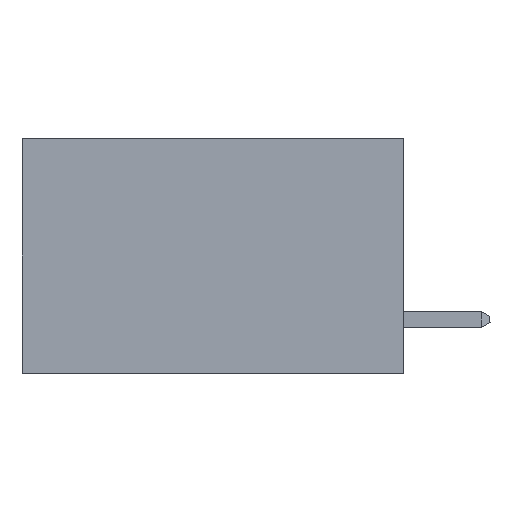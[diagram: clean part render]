
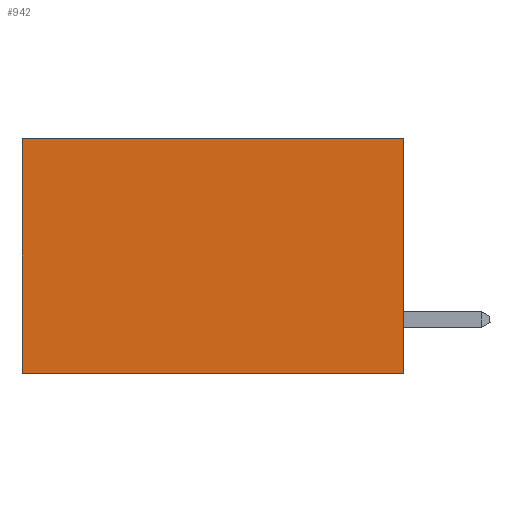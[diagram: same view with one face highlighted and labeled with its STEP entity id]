
A CAD part, left-side view. The second image highlights one B-rep face of the part: STEP entity #942.
In plain terms, the highlighted planar face has unit normal (-1, 0, 0).
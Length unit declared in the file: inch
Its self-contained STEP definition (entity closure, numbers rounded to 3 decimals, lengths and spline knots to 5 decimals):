
#180 = LINE ( 'NONE', #2519, #1146 ) ;
#942 = ADVANCED_FACE ( 'NONE', ( #18578 ), #19189, .F. ) ;
#993 = ORIENTED_EDGE ( 'NONE', *, *, #8523, .F. ) ;
#1146 = VECTOR ( 'NONE', #2720, 39.37008 ) ;
#1188 = VECTOR ( 'NONE', #8914, 39.37008 ) ;
#2519 = CARTESIAN_POINT ( 'NONE',  ( 0.2875, 0.6, 0. ) ) ;
#2554 = DIRECTION ( 'NONE',  ( 0., 1., 0. ) ) ;
#2698 = CARTESIAN_POINT ( 'NONE',  ( 0.2875, 0., 0. ) ) ;
#2720 = DIRECTION ( 'NONE',  ( 0., 0., -1. ) ) ;
#2776 = AXIS2_PLACEMENT_3D ( 'NONE', #10465, #11907, #9005 ) ;
#3345 = CARTESIAN_POINT ( 'NONE',  ( 0.2875, 0., 0. ) ) ;
#3592 = LINE ( 'NONE', #15604, #12800 ) ;
#4766 = EDGE_CURVE ( 'NONE', #13342, #5746, #180, .T. ) ;
#5746 = VERTEX_POINT ( 'NONE', #13239 ) ;
#8131 = CARTESIAN_POINT ( 'NONE',  ( 0.2875, 0.6, 0. ) ) ;
#8229 = LINE ( 'NONE', #8392, #11760 ) ;
#8392 = CARTESIAN_POINT ( 'NONE',  ( 0.2875, 0., 0. ) ) ;
#8523 = EDGE_CURVE ( 'NONE', #9525, #9038, #15133, .T. ) ;
#8914 = DIRECTION ( 'NONE',  ( 0., 0., -1. ) ) ;
#9005 = DIRECTION ( 'NONE',  ( 0., 0., -1. ) ) ;
#9038 = VERTEX_POINT ( 'NONE', #16742 ) ;
#9525 = VERTEX_POINT ( 'NONE', #3345 ) ;
#10369 = EDGE_CURVE ( 'NONE', #9525, #13342, #8229, .T. ) ;
#10465 = CARTESIAN_POINT ( 'NONE',  ( 0.2875, 0., 0. ) ) ;
#11164 = ORIENTED_EDGE ( 'NONE', *, *, #10369, .T. ) ;
#11349 = DIRECTION ( 'NONE',  ( 0., 1., 0. ) ) ;
#11760 = VECTOR ( 'NONE', #2554, 39.37008 ) ;
#11907 = DIRECTION ( 'NONE',  ( 1., 0., 0. ) ) ;
#12800 = VECTOR ( 'NONE', #11349, 39.37008 ) ;
#13239 = CARTESIAN_POINT ( 'NONE',  ( 0.2875, 0.6, -0.37 ) ) ;
#13342 = VERTEX_POINT ( 'NONE', #8131 ) ;
#15133 = LINE ( 'NONE', #2698, #1188 ) ;
#15321 = EDGE_LOOP ( 'NONE', ( #18373, #19346, #993, #11164 ) ) ;
#15604 = CARTESIAN_POINT ( 'NONE',  ( 0.2875, 0., -0.37 ) ) ;
#16742 = CARTESIAN_POINT ( 'NONE',  ( 0.2875, 0., -0.37 ) ) ;
#17082 = EDGE_CURVE ( 'NONE', #9038, #5746, #3592, .T. ) ;
#18373 = ORIENTED_EDGE ( 'NONE', *, *, #4766, .T. ) ;
#18578 = FACE_OUTER_BOUND ( 'NONE', #15321, .T. ) ;
#19189 = PLANE ( 'NONE',  #2776 ) ;
#19346 = ORIENTED_EDGE ( 'NONE', *, *, #17082, .F. ) ;
